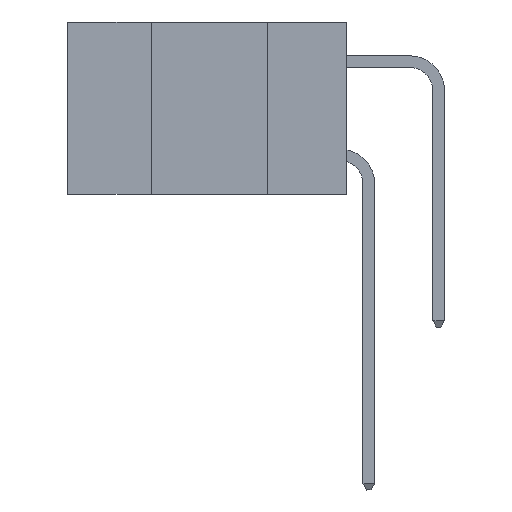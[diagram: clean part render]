
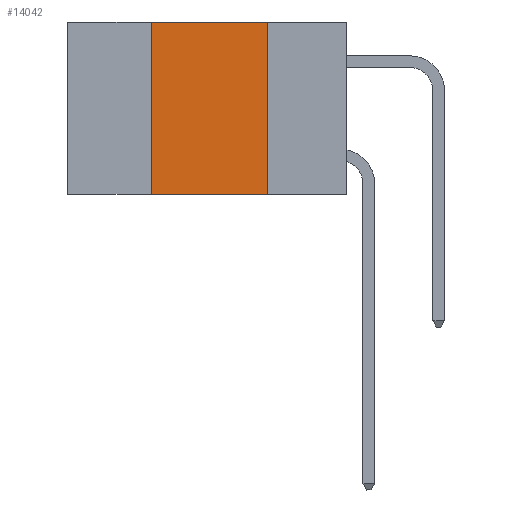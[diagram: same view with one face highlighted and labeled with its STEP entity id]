
A CAD part, left-side view. The second image highlights one B-rep face of the part: STEP entity #14042.
In plain terms, the highlighted planar face has unit normal (-1, 0, 0).
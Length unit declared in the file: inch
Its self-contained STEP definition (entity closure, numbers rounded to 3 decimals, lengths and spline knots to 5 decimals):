
#375 = ORIENTED_EDGE ( 'NONE', *, *, #895, .F. ) ;
#895 = EDGE_CURVE ( 'NONE', #12460, #15247, #8928, .T. ) ;
#1895 = DIRECTION ( 'NONE',  ( 0., 0., 1. ) ) ;
#1941 = CARTESIAN_POINT ( 'NONE',  ( 0., 0.17, -0.37 ) ) ;
#2630 = VERTEX_POINT ( 'NONE', #11897 ) ;
#2984 = ORIENTED_EDGE ( 'NONE', *, *, #12022, .F. ) ;
#3569 = PLANE ( 'NONE',  #6162 ) ;
#3803 = LINE ( 'NONE', #10310, #4367 ) ;
#4367 = VECTOR ( 'NONE', #12715, 39.37008 ) ;
#5738 = VECTOR ( 'NONE', #10759, 39.37008 ) ;
#6162 = AXIS2_PLACEMENT_3D ( 'NONE', #12013, #10894, #13227 ) ;
#6207 = CARTESIAN_POINT ( 'NONE',  ( 0., 0.17, 0. ) ) ;
#6835 = CARTESIAN_POINT ( 'NONE',  ( 0., 0.6, 0. ) ) ;
#7465 = VECTOR ( 'NONE', #1895, 39.37008 ) ;
#8293 = EDGE_CURVE ( 'NONE', #2630, #12460, #15048, .T. ) ;
#8529 = ORIENTED_EDGE ( 'NONE', *, *, #13137, .T. ) ;
#8734 = LINE ( 'NONE', #15747, #10821 ) ;
#8928 = LINE ( 'NONE', #6835, #5738 ) ;
#9311 = CARTESIAN_POINT ( 'NONE',  ( 0., 0.42, 0. ) ) ;
#9665 = DIRECTION ( 'NONE',  ( 0., 0., -1. ) ) ;
#10310 = CARTESIAN_POINT ( 'NONE',  ( 0., 0.6, -0.37 ) ) ;
#10759 = DIRECTION ( 'NONE',  ( 0., -1., 0. ) ) ;
#10821 = VECTOR ( 'NONE', #9665, 39.37008 ) ;
#10894 = DIRECTION ( 'NONE',  ( 1., 0., 0. ) ) ;
#11733 = CARTESIAN_POINT ( 'NONE',  ( 0., 0.42, 0. ) ) ;
#11897 = CARTESIAN_POINT ( 'NONE',  ( 0., 0.42, -0.37 ) ) ;
#11936 = VERTEX_POINT ( 'NONE', #1941 ) ;
#12013 = CARTESIAN_POINT ( 'NONE',  ( 0., 0.6, 0. ) ) ;
#12022 = EDGE_CURVE ( 'NONE', #15247, #11936, #8734, .T. ) ;
#12460 = VERTEX_POINT ( 'NONE', #11733 ) ;
#12654 = FACE_OUTER_BOUND ( 'NONE', #14756, .T. ) ;
#12715 = DIRECTION ( 'NONE',  ( 0., -1., 0. ) ) ;
#13137 = EDGE_CURVE ( 'NONE', #2630, #11936, #3803, .T. ) ;
#13227 = DIRECTION ( 'NONE',  ( 0., 0., -1. ) ) ;
#14042 = ADVANCED_FACE ( 'NONE', ( #12654 ), #3569, .F. ) ;
#14428 = ORIENTED_EDGE ( 'NONE', *, *, #8293, .F. ) ;
#14756 = EDGE_LOOP ( 'NONE', ( #2984, #375, #14428, #8529 ) ) ;
#15048 = LINE ( 'NONE', #9311, #7465 ) ;
#15247 = VERTEX_POINT ( 'NONE', #6207 ) ;
#15747 = CARTESIAN_POINT ( 'NONE',  ( 0., 0.17, 0. ) ) ;
